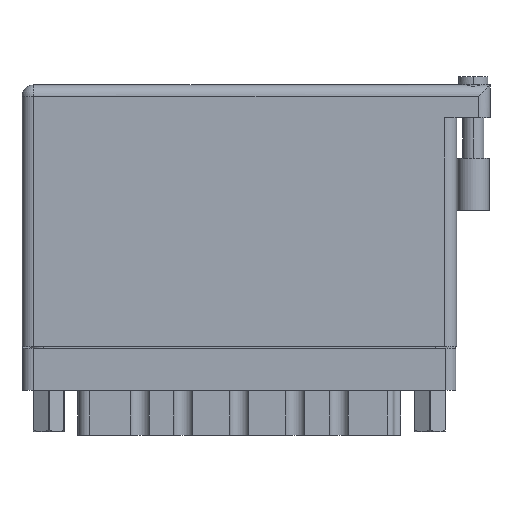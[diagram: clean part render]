
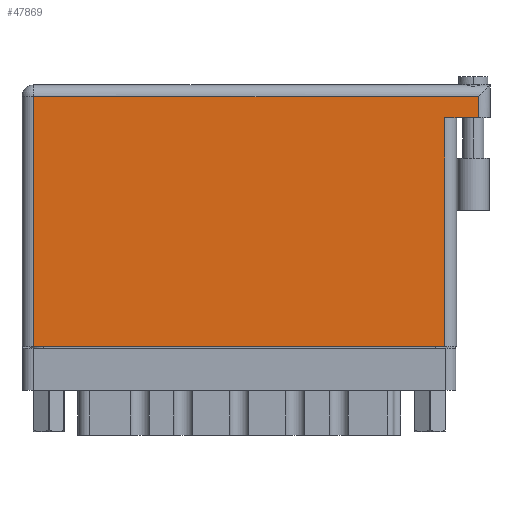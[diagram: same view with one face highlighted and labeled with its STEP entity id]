
A CAD part, front view. The second image highlights one B-rep face of the part: STEP entity #47869.
In plain terms, the highlighted face is planar.
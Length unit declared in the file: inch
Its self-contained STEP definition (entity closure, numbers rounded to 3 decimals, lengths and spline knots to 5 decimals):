
#264 = VERTEX_POINT ( 'NONE', #29028 ) ;
#1543 = EDGE_CURVE ( 'NONE', #36872, #22963, #57916, .T. ) ;
#1818 = VERTEX_POINT ( 'NONE', #35240 ) ;
#2023 = VECTOR ( 'NONE', #55509, 39.37008 ) ;
#2941 = DIRECTION ( 'NONE',  ( 0., 1., 0. ) ) ;
#6744 = CARTESIAN_POINT ( 'NONE',  ( 0.07, 0., 0. ) ) ;
#8525 = LINE ( 'NONE', #30644, #22788 ) ;
#10060 = ORIENTED_EDGE ( 'NONE', *, *, #1543, .F. ) ;
#11074 = EDGE_CURVE ( 'NONE', #1818, #31611, #56305, .T. ) ;
#11692 = LINE ( 'NONE', #6744, #2023 ) ;
#13411 = ORIENTED_EDGE ( 'NONE', *, *, #28278, .T. ) ;
#13893 = LINE ( 'NONE', #36599, #32638 ) ;
#14149 = EDGE_LOOP ( 'NONE', ( #13411, #41892, #10060, #42612, #28742, #22969 ) ) ;
#16801 = EDGE_CURVE ( 'NONE', #264, #22963, #13893, .T. ) ;
#17152 = DIRECTION ( 'NONE',  ( -1., 0., 0. ) ) ;
#17279 = CARTESIAN_POINT ( 'NONE',  ( 2.73, 1.566, 0. ) ) ;
#19576 = EDGE_CURVE ( 'NONE', #36872, #1818, #55782, .T. ) ;
#20650 = CARTESIAN_POINT ( 'NONE',  ( 0., 1.496, 0. ) ) ;
#21830 = CARTESIAN_POINT ( 'NONE',  ( 2.73, 1.369, 0. ) ) ;
#22201 = CARTESIAN_POINT ( 'NONE',  ( 0.07, 0., 0. ) ) ;
#22788 = VECTOR ( 'NONE', #36054, 39.37008 ) ;
#22963 = VERTEX_POINT ( 'NONE', #59256 ) ;
#22969 = ORIENTED_EDGE ( 'NONE', *, *, #25293, .T. ) ;
#24260 = VERTEX_POINT ( 'NONE', #22201 ) ;
#25293 = EDGE_CURVE ( 'NONE', #31611, #24260, #11692, .T. ) ;
#25354 = CARTESIAN_POINT ( 'NONE',  ( 0.07, 1.496, 0. ) ) ;
#28278 = EDGE_CURVE ( 'NONE', #24260, #264, #8525, .T. ) ;
#28742 = ORIENTED_EDGE ( 'NONE', *, *, #11074, .T. ) ;
#29028 = CARTESIAN_POINT ( 'NONE',  ( 2.53, 0., 0. ) ) ;
#30644 = CARTESIAN_POINT ( 'NONE',  ( 0., 0., 0. ) ) ;
#30891 = DIRECTION ( 'NONE',  ( -1., 0., 0. ) ) ;
#30979 = CARTESIAN_POINT ( 'NONE',  ( 0., 1.566, 0. ) ) ;
#31183 = DIRECTION ( 'NONE',  ( 0., 0., -1. ) ) ;
#31611 = VERTEX_POINT ( 'NONE', #25354 ) ;
#32191 = AXIS2_PLACEMENT_3D ( 'NONE', #30979, #31183, #17152 ) ;
#32638 = VECTOR ( 'NONE', #2941, 39.37008 ) ;
#35240 = CARTESIAN_POINT ( 'NONE',  ( 2.73, 1.496, 0. ) ) ;
#36054 = DIRECTION ( 'NONE',  ( 1., 0., 0. ) ) ;
#36599 = CARTESIAN_POINT ( 'NONE',  ( 2.53, 1.369, 0. ) ) ;
#36863 = VECTOR ( 'NONE', #38879, 39.37008 ) ;
#36872 = VERTEX_POINT ( 'NONE', #21830 ) ;
#38872 = CARTESIAN_POINT ( 'NONE',  ( 2.8, 1.369, 0. ) ) ;
#38879 = DIRECTION ( 'NONE',  ( -1., 0., 0. ) ) ;
#40696 = VECTOR ( 'NONE', #30891, 39.37008 ) ;
#41892 = ORIENTED_EDGE ( 'NONE', *, *, #16801, .T. ) ;
#42612 = ORIENTED_EDGE ( 'NONE', *, *, #19576, .T. ) ;
#43115 = VECTOR ( 'NONE', #60393, 39.37008 ) ;
#45474 = PLANE ( 'NONE',  #32191 ) ;
#47869 = ADVANCED_FACE ( 'NONE', ( #49438 ), #45474, .F. ) ;
#49438 = FACE_OUTER_BOUND ( 'NONE', #14149, .T. ) ;
#55509 = DIRECTION ( 'NONE',  ( 0., -1., 0. ) ) ;
#55782 = LINE ( 'NONE', #17279, #43115 ) ;
#56305 = LINE ( 'NONE', #20650, #36863 ) ;
#57916 = LINE ( 'NONE', #38872, #40696 ) ;
#59256 = CARTESIAN_POINT ( 'NONE',  ( 2.53, 1.369, 0. ) ) ;
#60393 = DIRECTION ( 'NONE',  ( 0., 1., 0. ) ) ;
